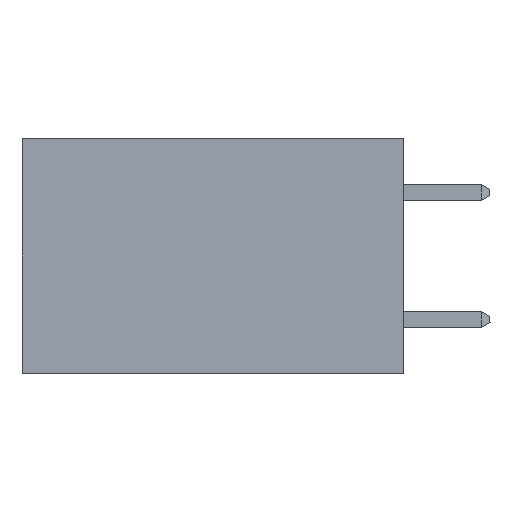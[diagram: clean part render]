
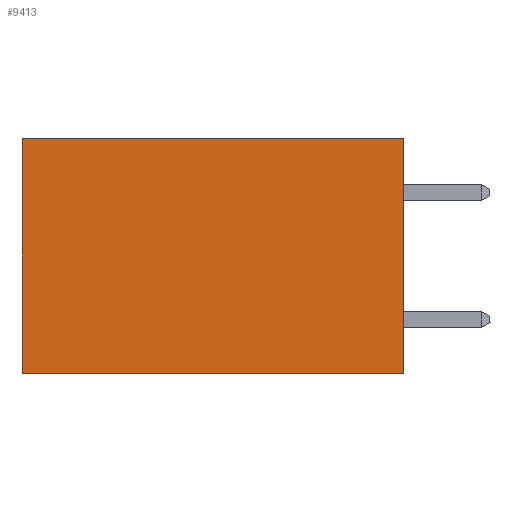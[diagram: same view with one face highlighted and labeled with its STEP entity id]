
A CAD part, left-side view. The second image highlights one B-rep face of the part: STEP entity #9413.
In plain terms, the highlighted planar face has unit normal (-1, 0, 0).
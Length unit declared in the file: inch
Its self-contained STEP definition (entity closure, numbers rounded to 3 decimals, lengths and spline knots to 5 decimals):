
#1355 = CARTESIAN_POINT ( 'NONE',  ( 0.2875, 0.6, 0. ) ) ;
#1623 = ORIENTED_EDGE ( 'NONE', *, *, #11007, .T. ) ;
#3828 = FACE_OUTER_BOUND ( 'NONE', #24973, .T. ) ;
#3833 = AXIS2_PLACEMENT_3D ( 'NONE', #21071, #9253, #13224 ) ;
#5200 = DIRECTION ( 'NONE',  ( 0., 1., 0. ) ) ;
#5858 = ORIENTED_EDGE ( 'NONE', *, *, #15812, .F. ) ;
#5908 = VECTOR ( 'NONE', #6599, 39.37008 ) ;
#6599 = DIRECTION ( 'NONE',  ( 0., 1., 0. ) ) ;
#9243 = ORIENTED_EDGE ( 'NONE', *, *, #16595, .T. ) ;
#9253 = DIRECTION ( 'NONE',  ( 1., 0., 0. ) ) ;
#9413 = ADVANCED_FACE ( 'NONE', ( #3828 ), #25038, .F. ) ;
#9630 = LINE ( 'NONE', #1355, #11470 ) ;
#10330 = VERTEX_POINT ( 'NONE', #16254 ) ;
#10990 = CARTESIAN_POINT ( 'NONE',  ( 0.2875, 0., -0.37 ) ) ;
#11007 = EDGE_CURVE ( 'NONE', #11355, #10330, #11099, .T. ) ;
#11099 = LINE ( 'NONE', #18332, #5908 ) ;
#11226 = ORIENTED_EDGE ( 'NONE', *, *, #21403, .F. ) ;
#11355 = VERTEX_POINT ( 'NONE', #15273 ) ;
#11470 = VECTOR ( 'NONE', #24806, 39.37008 ) ;
#11516 = CARTESIAN_POINT ( 'NONE',  ( 0.2875, 0., -0.37 ) ) ;
#13224 = DIRECTION ( 'NONE',  ( 0., 0., -1. ) ) ;
#15273 = CARTESIAN_POINT ( 'NONE',  ( 0.2875, 0., 0. ) ) ;
#15544 = CARTESIAN_POINT ( 'NONE',  ( 0.2875, 0., 0. ) ) ;
#15812 = EDGE_CURVE ( 'NONE', #21913, #24056, #16095, .T. ) ;
#16095 = LINE ( 'NONE', #10990, #23227 ) ;
#16254 = CARTESIAN_POINT ( 'NONE',  ( 0.2875, 0.6, 0. ) ) ;
#16595 = EDGE_CURVE ( 'NONE', #10330, #24056, #9630, .T. ) ;
#17715 = DIRECTION ( 'NONE',  ( 0., 0., -1. ) ) ;
#18332 = CARTESIAN_POINT ( 'NONE',  ( 0.2875, 0., 0. ) ) ;
#20528 = VECTOR ( 'NONE', #17715, 39.37008 ) ;
#21071 = CARTESIAN_POINT ( 'NONE',  ( 0.2875, 0., 0. ) ) ;
#21403 = EDGE_CURVE ( 'NONE', #11355, #21913, #21424, .T. ) ;
#21424 = LINE ( 'NONE', #15544, #20528 ) ;
#21913 = VERTEX_POINT ( 'NONE', #11516 ) ;
#23227 = VECTOR ( 'NONE', #5200, 39.37008 ) ;
#23856 = CARTESIAN_POINT ( 'NONE',  ( 0.2875, 0.6, -0.37 ) ) ;
#24056 = VERTEX_POINT ( 'NONE', #23856 ) ;
#24806 = DIRECTION ( 'NONE',  ( 0., 0., -1. ) ) ;
#24973 = EDGE_LOOP ( 'NONE', ( #9243, #5858, #11226, #1623 ) ) ;
#25038 = PLANE ( 'NONE',  #3833 ) ;
